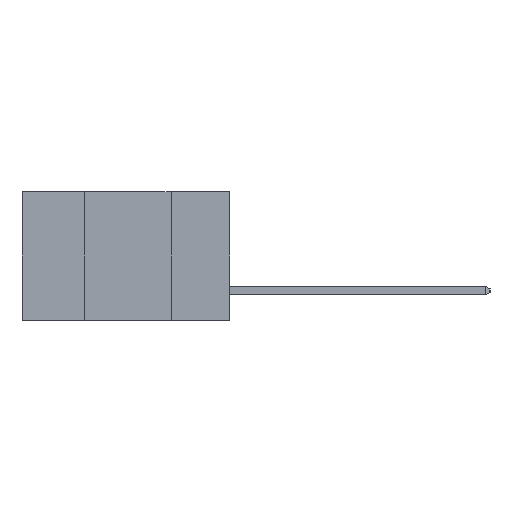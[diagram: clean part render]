
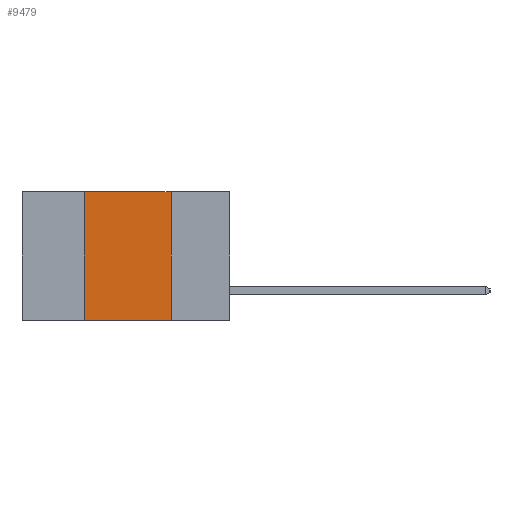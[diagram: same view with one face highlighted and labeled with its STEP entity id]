
A CAD part, left-side view. The second image highlights one B-rep face of the part: STEP entity #9479.
In plain terms, the highlighted planar face has unit normal (-1, 0, 0).
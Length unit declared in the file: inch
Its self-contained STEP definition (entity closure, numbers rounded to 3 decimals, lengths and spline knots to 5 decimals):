
#408 = PLANE ( 'NONE',  #9957 ) ;
#1762 = DIRECTION ( 'NONE',  ( 1., 0., 0. ) ) ;
#2160 = EDGE_CURVE ( 'NONE', #7335, #10892, #5563, .T. ) ;
#2269 = LINE ( 'NONE', #16114, #3740 ) ;
#2287 = ORIENTED_EDGE ( 'NONE', *, *, #13517, .F. ) ;
#2455 = VERTEX_POINT ( 'NONE', #16130 ) ;
#2606 = CARTESIAN_POINT ( 'NONE',  ( 0., 0.42, 0. ) ) ;
#2829 = EDGE_CURVE ( 'NONE', #2455, #14617, #15963, .T. ) ;
#3740 = VECTOR ( 'NONE', #8120, 39.37008 ) ;
#4823 = DIRECTION ( 'NONE',  ( 0., 0., -1. ) ) ;
#4856 = CARTESIAN_POINT ( 'NONE',  ( 0., 0.17, 0. ) ) ;
#5050 = CARTESIAN_POINT ( 'NONE',  ( 0., 0.17, 0. ) ) ;
#5221 = FACE_OUTER_BOUND ( 'NONE', #7178, .T. ) ;
#5292 = DIRECTION ( 'NONE',  ( 0., -1., 0. ) ) ;
#5520 = EDGE_CURVE ( 'NONE', #2455, #10892, #7390, .T. ) ;
#5563 = LINE ( 'NONE', #5050, #5985 ) ;
#5985 = VECTOR ( 'NONE', #4823, 39.37008 ) ;
#7178 = EDGE_LOOP ( 'NONE', ( #8205, #2287, #15789, #10811 ) ) ;
#7335 = VERTEX_POINT ( 'NONE', #4856 ) ;
#7390 = LINE ( 'NONE', #15048, #14049 ) ;
#7911 = DIRECTION ( 'NONE',  ( 0., 0., 1. ) ) ;
#8120 = DIRECTION ( 'NONE',  ( 0., -1., 0. ) ) ;
#8205 = ORIENTED_EDGE ( 'NONE', *, *, #2160, .F. ) ;
#8854 = VECTOR ( 'NONE', #7911, 39.37008 ) ;
#8986 = CARTESIAN_POINT ( 'NONE',  ( 0., 0.17, -0.37 ) ) ;
#9479 = ADVANCED_FACE ( 'NONE', ( #5221 ), #408, .F. ) ;
#9957 = AXIS2_PLACEMENT_3D ( 'NONE', #16324, #1762, #11022 ) ;
#10811 = ORIENTED_EDGE ( 'NONE', *, *, #5520, .T. ) ;
#10892 = VERTEX_POINT ( 'NONE', #8986 ) ;
#11022 = DIRECTION ( 'NONE',  ( 0., 0., -1. ) ) ;
#11720 = CARTESIAN_POINT ( 'NONE',  ( 0., 0.42, 0. ) ) ;
#13517 = EDGE_CURVE ( 'NONE', #14617, #7335, #2269, .T. ) ;
#14049 = VECTOR ( 'NONE', #5292, 39.37008 ) ;
#14617 = VERTEX_POINT ( 'NONE', #11720 ) ;
#15048 = CARTESIAN_POINT ( 'NONE',  ( 0., 0.6, -0.37 ) ) ;
#15789 = ORIENTED_EDGE ( 'NONE', *, *, #2829, .F. ) ;
#15963 = LINE ( 'NONE', #2606, #8854 ) ;
#16114 = CARTESIAN_POINT ( 'NONE',  ( 0., 0.6, 0. ) ) ;
#16130 = CARTESIAN_POINT ( 'NONE',  ( 0., 0.42, -0.37 ) ) ;
#16324 = CARTESIAN_POINT ( 'NONE',  ( 0., 0.6, 0. ) ) ;
